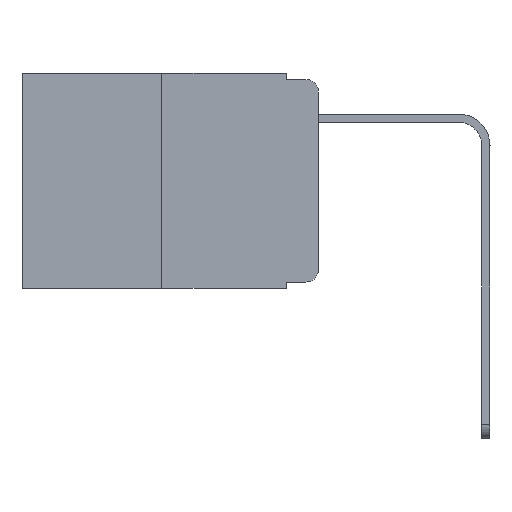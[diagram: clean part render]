
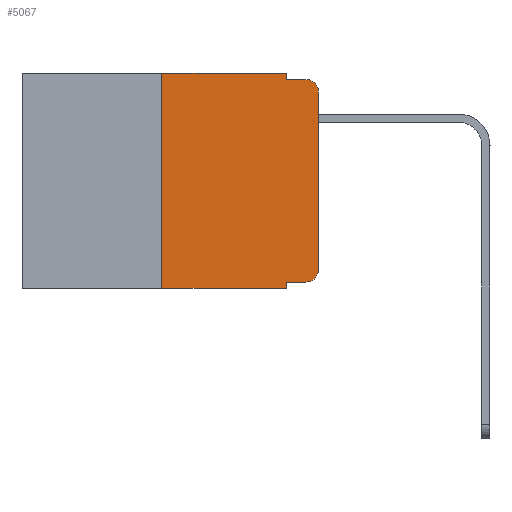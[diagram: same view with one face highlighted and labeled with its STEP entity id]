
A CAD part, left-side view. The second image highlights one B-rep face of the part: STEP entity #5067.
In plain terms, the highlighted planar face has unit normal (-1, 0, 0).
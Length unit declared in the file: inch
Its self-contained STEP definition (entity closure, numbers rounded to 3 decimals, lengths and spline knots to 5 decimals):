
#715 = ORIENTED_EDGE ( 'NONE', *, *, #8892, .F. ) ;
#785 = DIRECTION ( 'NONE',  ( 0., 0., 1. ) ) ;
#1092 = VECTOR ( 'NONE', #5701, 39.37008 ) ;
#1295 = VECTOR ( 'NONE', #18153, 39.37008 ) ;
#1768 = VERTEX_POINT ( 'NONE', #7578 ) ;
#2020 = LINE ( 'NONE', #19856, #18328 ) ;
#2042 = DIRECTION ( 'NONE',  ( -1., 0., 0. ) ) ;
#2116 = VERTEX_POINT ( 'NONE', #13258 ) ;
#2125 = AXIS2_PLACEMENT_3D ( 'NONE', #17696, #2042, #10631 ) ;
#2210 = VERTEX_POINT ( 'NONE', #9848 ) ;
#2437 = FACE_OUTER_BOUND ( 'NONE', #14632, .T. ) ;
#2500 = CARTESIAN_POINT ( 'NONE',  ( 0., 0.473, 0. ) ) ;
#2531 = DIRECTION ( 'NONE',  ( 0., 0., -1. ) ) ;
#2716 = LINE ( 'NONE', #14892, #19313 ) ;
#2832 = DIRECTION ( 'NONE',  ( 0., 0., -1. ) ) ;
#2905 = CARTESIAN_POINT ( 'NONE',  ( 0., 0.051, 0. ) ) ;
#3308 = VECTOR ( 'NONE', #785, 39.37008 ) ;
#3908 = VERTEX_POINT ( 'NONE', #17100 ) ;
#4249 = CARTESIAN_POINT ( 'NONE',  ( 0., 0.473, -0.343 ) ) ;
#4345 = DIRECTION ( 'NONE',  ( -1., 0., 0. ) ) ;
#4393 = DIRECTION ( 'NONE',  ( 0., -1., 0. ) ) ;
#5067 = ADVANCED_FACE ( 'NONE', ( #2437 ), #6516, .F. ) ;
#5211 = CARTESIAN_POINT ( 'NONE',  ( 0., 0.051, 0. ) ) ;
#5560 = EDGE_CURVE ( 'NONE', #3908, #16197, #10574, .T. ) ;
#5574 = EDGE_CURVE ( 'NONE', #12675, #19716, #15159, .T. ) ;
#5701 = DIRECTION ( 'NONE',  ( 0., 0., -1. ) ) ;
#6516 = PLANE ( 'NONE',  #8674 ) ;
#6749 = CARTESIAN_POINT ( 'NONE',  ( 0., 0.473, 0. ) ) ;
#6759 = CARTESIAN_POINT ( 'NONE',  ( 0., 0., 0. ) ) ;
#7309 = CARTESIAN_POINT ( 'NONE',  ( 0., 0.02, -0.333 ) ) ;
#7578 = CARTESIAN_POINT ( 'NONE',  ( 0., 0.051, -0.333 ) ) ;
#7678 = VECTOR ( 'NONE', #2832, 39.37008 ) ;
#7689 = CARTESIAN_POINT ( 'NONE',  ( 0., 0.051, -0.343 ) ) ;
#7914 = ORIENTED_EDGE ( 'NONE', *, *, #8682, .F. ) ;
#8549 = ORIENTED_EDGE ( 'NONE', *, *, #20531, .T. ) ;
#8674 = AXIS2_PLACEMENT_3D ( 'NONE', #6749, #15560, #17013 ) ;
#8682 = EDGE_CURVE ( 'NONE', #2210, #19624, #2020, .T. ) ;
#8892 = EDGE_CURVE ( 'NONE', #16197, #2210, #18588, .T. ) ;
#8941 = ORIENTED_EDGE ( 'NONE', *, *, #9917, .F. ) ;
#9426 = ORIENTED_EDGE ( 'NONE', *, *, #5574, .T. ) ;
#9741 = CIRCLE ( 'NONE', #10649, 0.02 ) ;
#9742 = ORIENTED_EDGE ( 'NONE', *, *, #11069, .T. ) ;
#9848 = CARTESIAN_POINT ( 'NONE',  ( 0., 0.051, -0.01 ) ) ;
#9917 = EDGE_CURVE ( 'NONE', #12675, #3908, #19887, .T. ) ;
#9927 = ORIENTED_EDGE ( 'NONE', *, *, #11966, .T. ) ;
#10547 = CIRCLE ( 'NONE', #2125, 0.02 ) ;
#10574 = LINE ( 'NONE', #2500, #1295 ) ;
#10631 = DIRECTION ( 'NONE',  ( 0., 0., -1. ) ) ;
#10649 = AXIS2_PLACEMENT_3D ( 'NONE', #15884, #4345, #2531 ) ;
#10673 = CARTESIAN_POINT ( 'NONE',  ( 0., 0.25, -0.343 ) ) ;
#11069 = EDGE_CURVE ( 'NONE', #1768, #16411, #2716, .T. ) ;
#11130 = CARTESIAN_POINT ( 'NONE',  ( 0., 0., -0.313 ) ) ;
#11143 = CARTESIAN_POINT ( 'NONE',  ( 0., 0.25, 0. ) ) ;
#11504 = ORIENTED_EDGE ( 'NONE', *, *, #5560, .F. ) ;
#11709 = DIRECTION ( 'NONE',  ( 0., -1., 0. ) ) ;
#11923 = ORIENTED_EDGE ( 'NONE', *, *, #17191, .T. ) ;
#11966 = EDGE_CURVE ( 'NONE', #16411, #15931, #10547, .T. ) ;
#12675 = VERTEX_POINT ( 'NONE', #10673 ) ;
#13258 = CARTESIAN_POINT ( 'NONE',  ( 0., 0., -0.03 ) ) ;
#13588 = DIRECTION ( 'NONE',  ( 0., 0., 1. ) ) ;
#13805 = ORIENTED_EDGE ( 'NONE', *, *, #20852, .F. ) ;
#14171 = CARTESIAN_POINT ( 'NONE',  ( 0., 0.02, -0.01 ) ) ;
#14632 = EDGE_LOOP ( 'NONE', ( #8549, #11923, #7914, #715, #11504, #8941, #9426, #13805, #9742, #9927 ) ) ;
#14660 = DIRECTION ( 'NONE',  ( 0., -1., 0. ) ) ;
#14706 = LINE ( 'NONE', #16027, #1092 ) ;
#14892 = CARTESIAN_POINT ( 'NONE',  ( 0., 0.051, -0.333 ) ) ;
#15159 = LINE ( 'NONE', #4249, #17642 ) ;
#15560 = DIRECTION ( 'NONE',  ( 1., 0., 0. ) ) ;
#15884 = CARTESIAN_POINT ( 'NONE',  ( 0., 0.02, -0.03 ) ) ;
#15931 = VERTEX_POINT ( 'NONE', #11130 ) ;
#16027 = CARTESIAN_POINT ( 'NONE',  ( 0., 0.051, 0. ) ) ;
#16197 = VERTEX_POINT ( 'NONE', #5211 ) ;
#16411 = VERTEX_POINT ( 'NONE', #7309 ) ;
#17013 = DIRECTION ( 'NONE',  ( 0., 0., -1. ) ) ;
#17100 = CARTESIAN_POINT ( 'NONE',  ( 0., 0.25, 0. ) ) ;
#17191 = EDGE_CURVE ( 'NONE', #2116, #19624, #9741, .T. ) ;
#17642 = VECTOR ( 'NONE', #4393, 39.37008 ) ;
#17696 = CARTESIAN_POINT ( 'NONE',  ( 0., 0.02, -0.313 ) ) ;
#18153 = DIRECTION ( 'NONE',  ( 0., -1., 0. ) ) ;
#18328 = VECTOR ( 'NONE', #14660, 39.37008 ) ;
#18588 = LINE ( 'NONE', #2905, #7678 ) ;
#19313 = VECTOR ( 'NONE', #11709, 39.37008 ) ;
#19624 = VERTEX_POINT ( 'NONE', #14171 ) ;
#19716 = VERTEX_POINT ( 'NONE', #7689 ) ;
#19856 = CARTESIAN_POINT ( 'NONE',  ( 0., 0.051, -0.01 ) ) ;
#19887 = LINE ( 'NONE', #11143, #3308 ) ;
#20531 = EDGE_CURVE ( 'NONE', #15931, #2116, #21568, .T. ) ;
#20852 = EDGE_CURVE ( 'NONE', #1768, #19716, #14706, .T. ) ;
#21568 = LINE ( 'NONE', #6759, #22117 ) ;
#22117 = VECTOR ( 'NONE', #13588, 39.37008 ) ;
